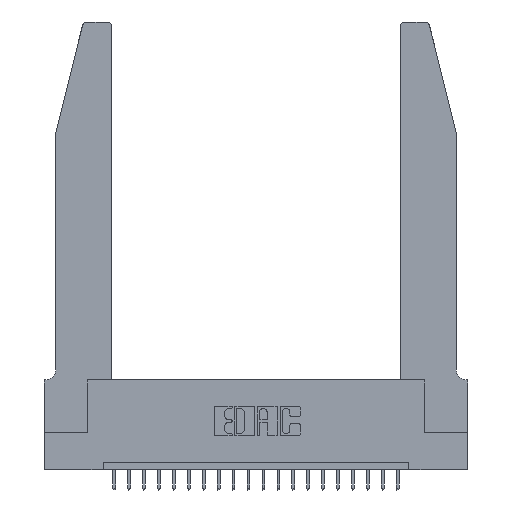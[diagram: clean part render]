
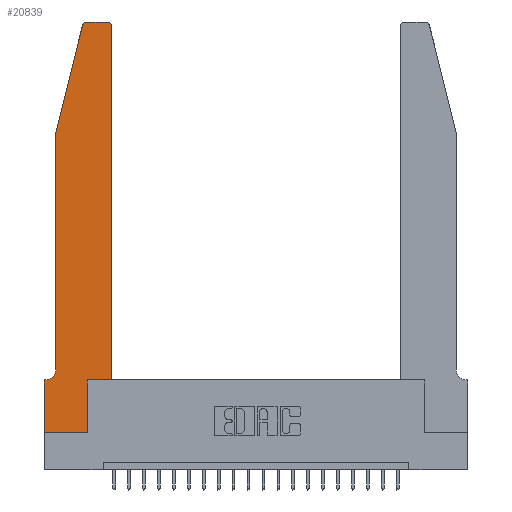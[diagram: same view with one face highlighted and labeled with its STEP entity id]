
A CAD part, top view. The second image highlights one B-rep face of the part: STEP entity #20839.
In plain terms, the highlighted planar face has unit normal (0, 0, 1).
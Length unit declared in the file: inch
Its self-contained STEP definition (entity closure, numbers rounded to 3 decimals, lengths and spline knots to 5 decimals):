
#465 = CARTESIAN_POINT ( 'NONE',  ( 0., 0.35, 0.37 ) ) ;
#590 = EDGE_CURVE ( 'NONE', #14883, #8059, #8663, .T. ) ;
#974 = VECTOR ( 'NONE', #16207, 39.37008 ) ;
#1021 = DIRECTION ( 'NONE',  ( 0., 1., 0. ) ) ;
#1159 = ORIENTED_EDGE ( 'NONE', *, *, #22738, .T. ) ;
#1764 = LINE ( 'NONE', #15806, #15076 ) ;
#1946 = VECTOR ( 'NONE', #11452, 39.37008 ) ;
#2000 = EDGE_CURVE ( 'NONE', #14814, #17273, #1764, .T. ) ;
#2067 = CARTESIAN_POINT ( 'NONE',  ( 0., 0., 0.37 ) ) ;
#2164 = EDGE_CURVE ( 'NONE', #5577, #14883, #19613, .T. ) ;
#2293 = CARTESIAN_POINT ( 'NONE',  ( 0., 0., 0.37 ) ) ;
#2297 = CARTESIAN_POINT ( 'NONE',  ( 0.0755, 2., 0.37 ) ) ;
#2376 = ORIENTED_EDGE ( 'NONE', *, *, #2000, .T. ) ;
#2448 = VERTEX_POINT ( 'NONE', #4810 ) ;
#2680 = AXIS2_PLACEMENT_3D ( 'NONE', #465, #7526, #21516 ) ;
#2817 = VECTOR ( 'NONE', #5700, 39.37008 ) ;
#3472 = CARTESIAN_POINT ( 'NONE',  ( 0.2865, 0.35, 0.37 ) ) ;
#4145 = PLANE ( 'NONE',  #2680 ) ;
#4448 = DIRECTION ( 'NONE',  ( 1., 0., 0. ) ) ;
#4687 = LINE ( 'NONE', #16752, #15880 ) ;
#4810 = CARTESIAN_POINT ( 'NONE',  ( 0.2865, 0., 0.37 ) ) ;
#5450 = EDGE_CURVE ( 'NONE', #14848, #2448, #4687, .T. ) ;
#5577 = VERTEX_POINT ( 'NONE', #19204 ) ;
#5700 = DIRECTION ( 'NONE',  ( -1., 0., 0. ) ) ;
#7507 = CARTESIAN_POINT ( 'NONE',  ( 0.0755, 0.42, 0.37 ) ) ;
#7526 = DIRECTION ( 'NONE',  ( 0., 0., 1. ) ) ;
#7578 = DIRECTION ( 'NONE',  ( -1., 0., 0. ) ) ;
#7677 = ORIENTED_EDGE ( 'NONE', *, *, #15698, .T. ) ;
#8059 = VERTEX_POINT ( 'NONE', #10331 ) ;
#8166 = ORIENTED_EDGE ( 'NONE', *, *, #5450, .T. ) ;
#8182 = VECTOR ( 'NONE', #20908, 39.37008 ) ;
#8328 = CARTESIAN_POINT ( 'NONE',  ( 0.4505, 2.72, 0.37 ) ) ;
#8663 = CIRCLE ( 'NONE', #21938, 0.07 ) ;
#8949 = DIRECTION ( 'NONE',  ( -1., 0., 0. ) ) ;
#9334 = CARTESIAN_POINT ( 'NONE',  ( 0.4505, 0.35, 0.37 ) ) ;
#9407 = CARTESIAN_POINT ( 'NONE',  ( 0.0755, 2., 0.37 ) ) ;
#9857 = ORIENTED_EDGE ( 'NONE', *, *, #17702, .T. ) ;
#10068 = CIRCLE ( 'NONE', #21524, 0.03 ) ;
#10331 = CARTESIAN_POINT ( 'NONE',  ( 0.0055, 0.35, 0.37 ) ) ;
#10425 = EDGE_CURVE ( 'NONE', #17166, #22660, #15144, .T. ) ;
#10770 = DIRECTION ( 'NONE',  ( 0., 1., 0. ) ) ;
#10799 = CARTESIAN_POINT ( 'NONE',  ( 0.2865, 0.35, 0.37 ) ) ;
#10966 = DIRECTION ( 'NONE',  ( 0., 0., -1. ) ) ;
#11117 = DIRECTION ( 'NONE',  ( 0., 0., 1. ) ) ;
#11408 = EDGE_CURVE ( 'NONE', #14603, #14814, #10068, .T. ) ;
#11452 = DIRECTION ( 'NONE',  ( -0.239, -0.971, 0. ) ) ;
#11486 = EDGE_CURVE ( 'NONE', #17866, #5577, #21832, .T. ) ;
#12057 = ORIENTED_EDGE ( 'NONE', *, *, #2164, .T. ) ;
#12874 = CARTESIAN_POINT ( 'NONE',  ( 0.284, 2.75, 0.37 ) ) ;
#12897 = ORIENTED_EDGE ( 'NONE', *, *, #11408, .T. ) ;
#13180 = VECTOR ( 'NONE', #10770, 39.37008 ) ;
#13519 = DIRECTION ( 'NONE',  ( 1., 0., 0. ) ) ;
#13951 = VERTEX_POINT ( 'NONE', #19938 ) ;
#13969 = ORIENTED_EDGE ( 'NONE', *, *, #10425, .T. ) ;
#14120 = DIRECTION ( 'NONE',  ( 1., 0., 0. ) ) ;
#14240 = CARTESIAN_POINT ( 'NONE',  ( 0.4205, 2.72, 0.37 ) ) ;
#14494 = VECTOR ( 'NONE', #1021, 39.37008 ) ;
#14602 = AXIS2_PLACEMENT_3D ( 'NONE', #15123, #20321, #4448 ) ;
#14603 = VERTEX_POINT ( 'NONE', #8328 ) ;
#14645 = CARTESIAN_POINT ( 'NONE',  ( 0.0755, 0.35, 0.37 ) ) ;
#14676 = ORIENTED_EDGE ( 'NONE', *, *, #590, .T. ) ;
#14814 = VERTEX_POINT ( 'NONE', #18174 ) ;
#14848 = VERTEX_POINT ( 'NONE', #2293 ) ;
#14883 = VERTEX_POINT ( 'NONE', #7507 ) ;
#14910 = ORIENTED_EDGE ( 'NONE', *, *, #11486, .T. ) ;
#15046 = LINE ( 'NONE', #22080, #14494 ) ;
#15076 = VECTOR ( 'NONE', #8949, 39.37008 ) ;
#15123 = CARTESIAN_POINT ( 'NONE',  ( 0.284, 2.72, 0.37 ) ) ;
#15144 = LINE ( 'NONE', #17218, #8182 ) ;
#15698 = EDGE_CURVE ( 'NONE', #8059, #13951, #21443, .T. ) ;
#15806 = CARTESIAN_POINT ( 'NONE',  ( 0.2605, 2.75, 0.37 ) ) ;
#15880 = VECTOR ( 'NONE', #13519, 39.37008 ) ;
#16207 = DIRECTION ( 'NONE',  ( 0., -1., 0. ) ) ;
#16275 = CARTESIAN_POINT ( 'NONE',  ( 0.0055, 0.42, 0.37 ) ) ;
#16332 = FACE_OUTER_BOUND ( 'NONE', #21699, .T. ) ;
#16752 = CARTESIAN_POINT ( 'NONE',  ( 0., 0., 0.37 ) ) ;
#16901 = VECTOR ( 'NONE', #18109, 39.37008 ) ;
#17166 = VERTEX_POINT ( 'NONE', #10799 ) ;
#17218 = CARTESIAN_POINT ( 'NONE',  ( 0.4505, 0.35, 0.37 ) ) ;
#17273 = VERTEX_POINT ( 'NONE', #12874 ) ;
#17334 = CARTESIAN_POINT ( 'NONE',  ( 0.25487, 2.72718, 0.37 ) ) ;
#17672 = EDGE_CURVE ( 'NONE', #2448, #17166, #19356, .T. ) ;
#17702 = EDGE_CURVE ( 'NONE', #13951, #14848, #17943, .T. ) ;
#17866 = VERTEX_POINT ( 'NONE', #17334 ) ;
#17943 = LINE ( 'NONE', #2067, #974 ) ;
#18109 = DIRECTION ( 'NONE',  ( 0., -1., 0. ) ) ;
#18174 = CARTESIAN_POINT ( 'NONE',  ( 0.4205, 2.75, 0.37 ) ) ;
#18290 = CIRCLE ( 'NONE', #14602, 0.03 ) ;
#19204 = CARTESIAN_POINT ( 'NONE',  ( 0.0755, 2., 0.37 ) ) ;
#19356 = LINE ( 'NONE', #3472, #13180 ) ;
#19613 = LINE ( 'NONE', #9407, #16901 ) ;
#19694 = EDGE_CURVE ( 'NONE', #22660, #14603, #15046, .T. ) ;
#19938 = CARTESIAN_POINT ( 'NONE',  ( 0., 0.35, 0.37 ) ) ;
#20321 = DIRECTION ( 'NONE',  ( 0., 0., 1. ) ) ;
#20422 = ORIENTED_EDGE ( 'NONE', *, *, #19694, .T. ) ;
#20839 = ADVANCED_FACE ( 'NONE', ( #16332 ), #4145, .T. ) ;
#20908 = DIRECTION ( 'NONE',  ( 1., 0., 0. ) ) ;
#21443 = LINE ( 'NONE', #14645, #2817 ) ;
#21516 = DIRECTION ( 'NONE',  ( 1., 0., 0. ) ) ;
#21524 = AXIS2_PLACEMENT_3D ( 'NONE', #14240, #11117, #14120 ) ;
#21699 = EDGE_LOOP ( 'NONE', ( #2376, #1159, #14910, #12057, #14676, #7677, #9857, #8166, #22210, #13969, #20422, #12897 ) ) ;
#21832 = LINE ( 'NONE', #2297, #1946 ) ;
#21938 = AXIS2_PLACEMENT_3D ( 'NONE', #16275, #10966, #7578 ) ;
#22080 = CARTESIAN_POINT ( 'NONE',  ( 0.4505, 0.35, 0.37 ) ) ;
#22210 = ORIENTED_EDGE ( 'NONE', *, *, #17672, .T. ) ;
#22660 = VERTEX_POINT ( 'NONE', #9334 ) ;
#22738 = EDGE_CURVE ( 'NONE', #17273, #17866, #18290, .T. ) ;
